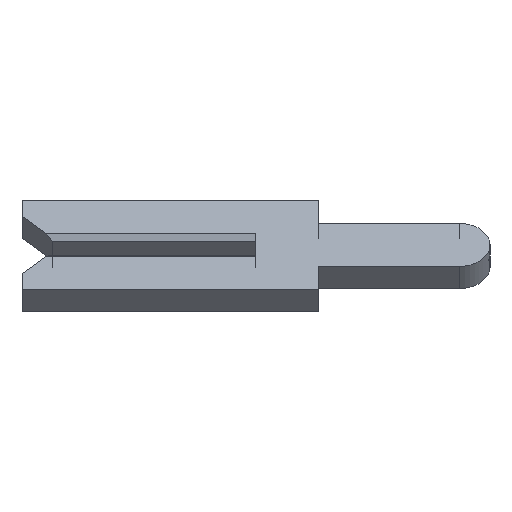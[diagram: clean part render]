
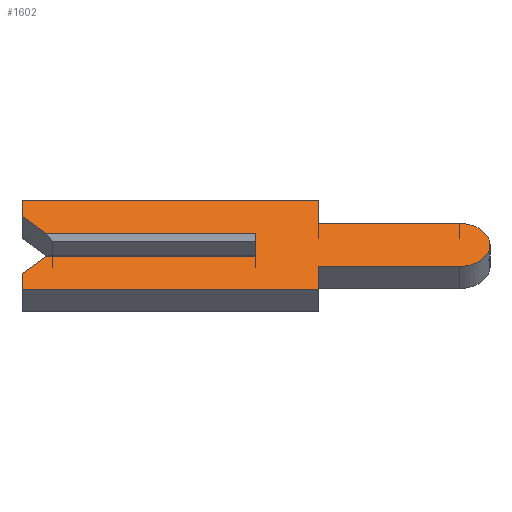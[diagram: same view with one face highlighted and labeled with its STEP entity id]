
A CAD part, left-side view. The second image highlights one B-rep face of the part: STEP entity #1602.
In plain terms, the highlighted face is planar.
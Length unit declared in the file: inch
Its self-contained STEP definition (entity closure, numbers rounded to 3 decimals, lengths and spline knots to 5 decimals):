
#2 = CARTESIAN_POINT ( 'NONE',  ( -0.01, -0.1305, 0. ) ) ;
#3 = EDGE_CURVE ( 'NONE', #1596, #1615, #205, .T. ) ;
#5 = VECTOR ( 'NONE', #547, 39.37008 ) ;
#7 = DIRECTION ( 'NONE',  ( 0., 0., 1. ) ) ;
#15 = DIRECTION ( 'NONE',  ( 0., 0., -1. ) ) ;
#30 = LINE ( 'NONE', #1359, #220 ) ;
#33 = CARTESIAN_POINT ( 'NONE',  ( -0.01, 0.15, 0.04 ) ) ;
#45 = CARTESIAN_POINT ( 'NONE',  ( -0.01, -0.04, 0.04 ) ) ;
#49 = LINE ( 'NONE', #119, #1502 ) ;
#82 = EDGE_CURVE ( 'NONE', #1313, #572, #844, .T. ) ;
#101 = EDGE_CURVE ( 'NONE', #1615, #696, #112, .T. ) ;
#107 = CARTESIAN_POINT ( 'NONE',  ( -0.01, -0.04, -0.0195 ) ) ;
#112 = CIRCLE ( 'NONE', #1019, 0.0195 ) ;
#117 = ORIENTED_EDGE ( 'NONE', *, *, #699, .F. ) ;
#119 = CARTESIAN_POINT ( 'NONE',  ( -0.01, 0.15, 0.01 ) ) ;
#123 = PLANE ( 'NONE',  #1554 ) ;
#126 = LINE ( 'NONE', #1096, #1622 ) ;
#170 = LINE ( 'NONE', #1223, #1063 ) ;
#180 = DIRECTION ( 'NONE',  ( 0., 0.707, 0.707 ) ) ;
#205 = LINE ( 'NONE', #1155, #713 ) ;
#211 = ORIENTED_EDGE ( 'NONE', *, *, #986, .F. ) ;
#220 = VECTOR ( 'NONE', #332, 39.37008 ) ;
#230 = VERTEX_POINT ( 'NONE', #1316 ) ;
#237 = DIRECTION ( 'NONE',  ( 0., -1., 0. ) ) ;
#244 = ORIENTED_EDGE ( 'NONE', *, *, #1135, .F. ) ;
#268 = ORIENTED_EDGE ( 'NONE', *, *, #1118, .T. ) ;
#327 = EDGE_LOOP ( 'NONE', ( #268, #211, #1629, #927, #609, #1266, #680, #1390, #1287, #776, #1130, #1591, #244, #117 ) ) ;
#332 = DIRECTION ( 'NONE',  ( 0., 1., 0. ) ) ;
#335 = LINE ( 'NONE', #752, #557 ) ;
#390 = CARTESIAN_POINT ( 'NONE',  ( -0.01, -0.1305, 0.0195 ) ) ;
#395 = VECTOR ( 'NONE', #764, 39.37008 ) ;
#447 = VERTEX_POINT ( 'NONE', #45 ) ;
#461 = DIRECTION ( 'NONE',  ( 0., -1., 0. ) ) ;
#468 = CARTESIAN_POINT ( 'NONE',  ( -0.01, 0.15, 0.026 ) ) ;
#472 = CARTESIAN_POINT ( 'NONE',  ( -0.01, 0.15, 0.04 ) ) ;
#478 = VERTEX_POINT ( 'NONE', #33 ) ;
#494 = CARTESIAN_POINT ( 'NONE',  ( -0.01, 0.15, -0.026 ) ) ;
#517 = VECTOR ( 'NONE', #1192, 39.37008 ) ;
#525 = DIRECTION ( 'NONE',  ( 0., 0., -1. ) ) ;
#547 = DIRECTION ( 'NONE',  ( 0., 0., 1. ) ) ;
#556 = CARTESIAN_POINT ( 'NONE',  ( -0.01, -0.1305, -0.0195 ) ) ;
#557 = VECTOR ( 'NONE', #1520, 39.37008 ) ;
#572 = VERTEX_POINT ( 'NONE', #1171 ) ;
#606 = CARTESIAN_POINT ( 'NONE',  ( -0.01, 0.15, -0.04 ) ) ;
#609 = ORIENTED_EDGE ( 'NONE', *, *, #82, .F. ) ;
#617 = DIRECTION ( 'NONE',  ( 0., -1., 0. ) ) ;
#666 = EDGE_CURVE ( 'NONE', #717, #230, #170, .T. ) ;
#671 = CARTESIAN_POINT ( 'NONE',  ( -0.01, 0., 0.0065 ) ) ;
#680 = ORIENTED_EDGE ( 'NONE', *, *, #1039, .F. ) ;
#696 = VERTEX_POINT ( 'NONE', #556 ) ;
#699 = EDGE_CURVE ( 'NONE', #883, #1371, #126, .T. ) ;
#713 = VECTOR ( 'NONE', #1416, 39.37008 ) ;
#717 = VERTEX_POINT ( 'NONE', #1356 ) ;
#752 = CARTESIAN_POINT ( 'NONE',  ( -0.01, -0.04, -0.04 ) ) ;
#764 = DIRECTION ( 'NONE',  ( 0., 1., 0. ) ) ;
#767 = EDGE_CURVE ( 'NONE', #696, #1451, #30, .T. ) ;
#768 = DIRECTION ( 'NONE',  ( 1., 0., 0. ) ) ;
#776 = ORIENTED_EDGE ( 'NONE', *, *, #3, .F. ) ;
#786 = CARTESIAN_POINT ( 'NONE',  ( -0.01, -0.1305, 0. ) ) ;
#829 = EDGE_CURVE ( 'NONE', #572, #717, #1603, .T. ) ;
#844 = LINE ( 'NONE', #494, #1046 ) ;
#883 = VERTEX_POINT ( 'NONE', #1094 ) ;
#894 = DIRECTION ( 'NONE',  ( 0., 0., -1. ) ) ;
#901 = CARTESIAN_POINT ( 'NONE',  ( -0.01, -0.04, 0.0195 ) ) ;
#927 = ORIENTED_EDGE ( 'NONE', *, *, #829, .F. ) ;
#966 = LINE ( 'NONE', #671, #1330 ) ;
#986 = EDGE_CURVE ( 'NONE', #230, #1406, #966, .T. ) ;
#994 = CARTESIAN_POINT ( 'NONE',  ( -0.01, 0.15, -0.04 ) ) ;
#1019 = AXIS2_PLACEMENT_3D ( 'NONE', #2, #768, #894 ) ;
#1037 = CARTESIAN_POINT ( 'NONE',  ( -0.01, -0.04, 0.04 ) ) ;
#1039 = EDGE_CURVE ( 'NONE', #1451, #1613, #335, .T. ) ;
#1046 = VECTOR ( 'NONE', #7, 39.37008 ) ;
#1063 = VECTOR ( 'NONE', #461, 39.37008 ) ;
#1082 = EDGE_CURVE ( 'NONE', #478, #447, #1582, .T. ) ;
#1094 = CARTESIAN_POINT ( 'NONE',  ( -0.01, 0.134, 0.01 ) ) ;
#1096 = CARTESIAN_POINT ( 'NONE',  ( -0.01, 0.1305, 0.0065 ) ) ;
#1108 = LINE ( 'NONE', #1037, #1334 ) ;
#1114 = CARTESIAN_POINT ( 'NONE',  ( -0.01, 0., 0.01 ) ) ;
#1118 = EDGE_CURVE ( 'NONE', #883, #1406, #49, .T. ) ;
#1130 = ORIENTED_EDGE ( 'NONE', *, *, #1577, .F. ) ;
#1135 = EDGE_CURVE ( 'NONE', #1371, #478, #1443, .T. ) ;
#1155 = CARTESIAN_POINT ( 'NONE',  ( -0.01, -0.04, 0.0195 ) ) ;
#1158 = CARTESIAN_POINT ( 'NONE',  ( -0.01, -0.04, -0.04 ) ) ;
#1171 = CARTESIAN_POINT ( 'NONE',  ( -0.01, 0.15, -0.026 ) ) ;
#1192 = DIRECTION ( 'NONE',  ( 0., -0.707, 0.707 ) ) ;
#1194 = VECTOR ( 'NONE', #237, 39.37008 ) ;
#1223 = CARTESIAN_POINT ( 'NONE',  ( -0.01, -0.1305, -0.01 ) ) ;
#1250 = EDGE_CURVE ( 'NONE', #1613, #1313, #1590, .T. ) ;
#1266 = ORIENTED_EDGE ( 'NONE', *, *, #1250, .F. ) ;
#1287 = ORIENTED_EDGE ( 'NONE', *, *, #101, .F. ) ;
#1313 = VERTEX_POINT ( 'NONE', #994 ) ;
#1316 = CARTESIAN_POINT ( 'NONE',  ( -0.01, 0., -0.01 ) ) ;
#1319 = DIRECTION ( 'NONE',  ( 0., 0., 1. ) ) ;
#1330 = VECTOR ( 'NONE', #1319, 39.37008 ) ;
#1334 = VECTOR ( 'NONE', #525, 39.37008 ) ;
#1356 = CARTESIAN_POINT ( 'NONE',  ( -0.01, 0.134, -0.01 ) ) ;
#1359 = CARTESIAN_POINT ( 'NONE',  ( -0.01, -0.04, -0.0195 ) ) ;
#1371 = VERTEX_POINT ( 'NONE', #468 ) ;
#1379 = CARTESIAN_POINT ( 'NONE',  ( -0.01, 0.15, 0.026 ) ) ;
#1390 = ORIENTED_EDGE ( 'NONE', *, *, #767, .F. ) ;
#1406 = VERTEX_POINT ( 'NONE', #1114 ) ;
#1415 = DIRECTION ( 'NONE',  ( 1., 0., 0. ) ) ;
#1416 = DIRECTION ( 'NONE',  ( 0., -1., 0. ) ) ;
#1443 = LINE ( 'NONE', #1379, #5 ) ;
#1451 = VERTEX_POINT ( 'NONE', #107 ) ;
#1502 = VECTOR ( 'NONE', #617, 39.37008 ) ;
#1520 = DIRECTION ( 'NONE',  ( 0., 0., -1. ) ) ;
#1551 = FACE_OUTER_BOUND ( 'NONE', #327, .T. ) ;
#1554 = AXIS2_PLACEMENT_3D ( 'NONE', #786, #1415, #15 ) ;
#1577 = EDGE_CURVE ( 'NONE', #447, #1596, #1108, .T. ) ;
#1582 = LINE ( 'NONE', #472, #1194 ) ;
#1590 = LINE ( 'NONE', #606, #395 ) ;
#1591 = ORIENTED_EDGE ( 'NONE', *, *, #1082, .F. ) ;
#1596 = VERTEX_POINT ( 'NONE', #901 ) ;
#1602 = ADVANCED_FACE ( 'NONE', ( #1551 ), #123, .F. ) ;
#1603 = LINE ( 'NONE', #1617, #517 ) ;
#1613 = VERTEX_POINT ( 'NONE', #1158 ) ;
#1615 = VERTEX_POINT ( 'NONE', #390 ) ;
#1617 = CARTESIAN_POINT ( 'NONE',  ( -0.01, 0.1305, -0.0065 ) ) ;
#1622 = VECTOR ( 'NONE', #180, 39.37008 ) ;
#1629 = ORIENTED_EDGE ( 'NONE', *, *, #666, .F. ) ;
